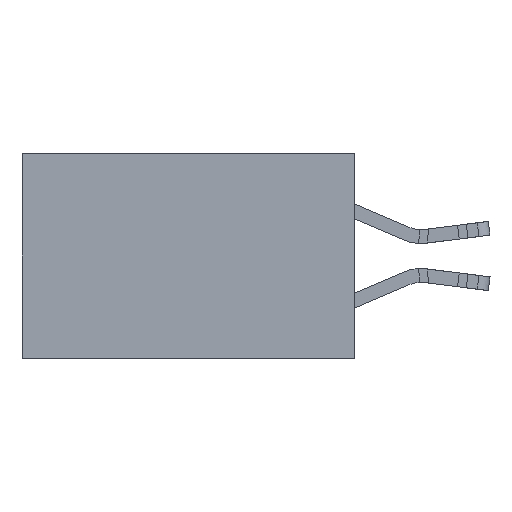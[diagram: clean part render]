
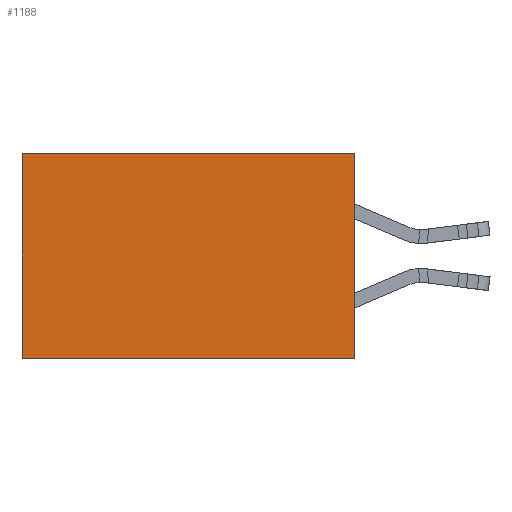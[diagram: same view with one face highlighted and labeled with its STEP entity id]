
A CAD part, left-side view. The second image highlights one B-rep face of the part: STEP entity #1188.
In plain terms, the highlighted planar face has unit normal (-1, 0, 0).
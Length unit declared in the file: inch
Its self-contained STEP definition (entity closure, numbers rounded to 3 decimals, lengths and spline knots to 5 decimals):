
#683 = CARTESIAN_POINT ( 'NONE',  ( 0.298, 0., 0. ) ) ;
#1160 = LINE ( 'NONE', #683, #7440 ) ;
#1188 = ADVANCED_FACE ( 'NONE', ( #2435 ), #17341, .F. ) ;
#2435 = FACE_OUTER_BOUND ( 'NONE', #4892, .T. ) ;
#2594 = VECTOR ( 'NONE', #20260, 39.37008 ) ;
#2660 = ORIENTED_EDGE ( 'NONE', *, *, #6855, .T. ) ;
#2883 = CARTESIAN_POINT ( 'NONE',  ( 0.298, 0.6, -0.37 ) ) ;
#3128 = DIRECTION ( 'NONE',  ( 0., 0., -1. ) ) ;
#3636 = CARTESIAN_POINT ( 'NONE',  ( 0.298, 0., 0. ) ) ;
#4662 = VERTEX_POINT ( 'NONE', #2883 ) ;
#4774 = VERTEX_POINT ( 'NONE', #5573 ) ;
#4892 = EDGE_LOOP ( 'NONE', ( #11554, #8090, #24573, #2660 ) ) ;
#5398 = DIRECTION ( 'NONE',  ( 1., 0., 0. ) ) ;
#5573 = CARTESIAN_POINT ( 'NONE',  ( 0.298, 0., 0. ) ) ;
#5758 = EDGE_CURVE ( 'NONE', #9013, #4662, #16451, .T. ) ;
#6167 = DIRECTION ( 'NONE',  ( 0., 1., 0. ) ) ;
#6855 = EDGE_CURVE ( 'NONE', #4774, #9013, #1160, .T. ) ;
#7440 = VECTOR ( 'NONE', #17277, 39.37008 ) ;
#8090 = ORIENTED_EDGE ( 'NONE', *, *, #11127, .F. ) ;
#9013 = VERTEX_POINT ( 'NONE', #28596 ) ;
#11127 = EDGE_CURVE ( 'NONE', #29475, #4662, #28908, .T. ) ;
#11554 = ORIENTED_EDGE ( 'NONE', *, *, #5758, .T. ) ;
#12127 = EDGE_CURVE ( 'NONE', #4774, #29475, #12582, .T. ) ;
#12582 = LINE ( 'NONE', #3636, #2594 ) ;
#15359 = CARTESIAN_POINT ( 'NONE',  ( 0.298, 0., 0. ) ) ;
#15488 = DIRECTION ( 'NONE',  ( 0., 0., -1. ) ) ;
#16451 = LINE ( 'NONE', #29645, #29021 ) ;
#16828 = AXIS2_PLACEMENT_3D ( 'NONE', #15359, #5398, #3128 ) ;
#17277 = DIRECTION ( 'NONE',  ( 0., 1., 0. ) ) ;
#17341 = PLANE ( 'NONE',  #16828 ) ;
#20260 = DIRECTION ( 'NONE',  ( 0., 0., -1. ) ) ;
#20418 = CARTESIAN_POINT ( 'NONE',  ( 0.298, 0., -0.37 ) ) ;
#24573 = ORIENTED_EDGE ( 'NONE', *, *, #12127, .F. ) ;
#27622 = CARTESIAN_POINT ( 'NONE',  ( 0.298, 0., -0.37 ) ) ;
#28596 = CARTESIAN_POINT ( 'NONE',  ( 0.298, 0.6, 0. ) ) ;
#28908 = LINE ( 'NONE', #27622, #29659 ) ;
#29021 = VECTOR ( 'NONE', #15488, 39.37008 ) ;
#29475 = VERTEX_POINT ( 'NONE', #20418 ) ;
#29645 = CARTESIAN_POINT ( 'NONE',  ( 0.298, 0.6, 0. ) ) ;
#29659 = VECTOR ( 'NONE', #6167, 39.37008 ) ;
